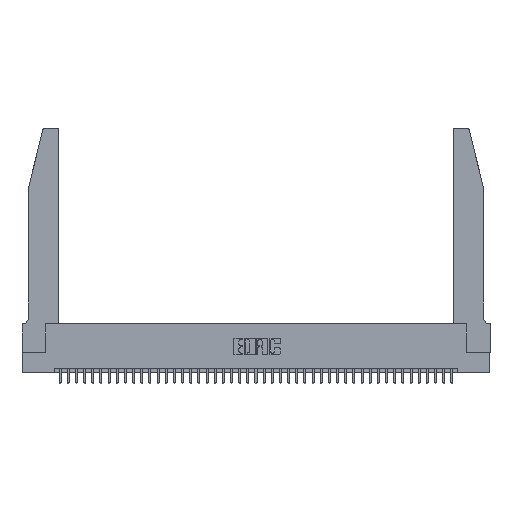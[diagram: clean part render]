
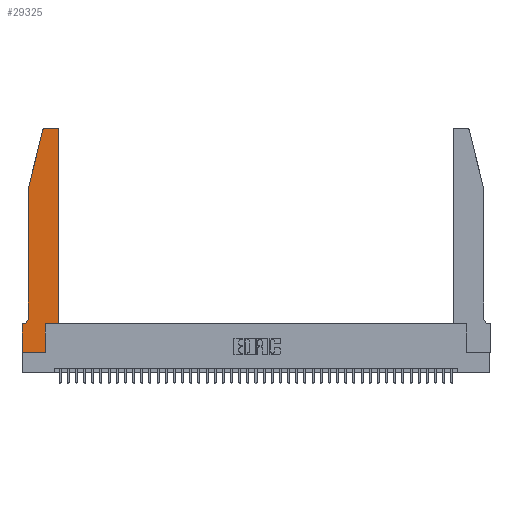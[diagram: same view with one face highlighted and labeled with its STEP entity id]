
A CAD part, top view. The second image highlights one B-rep face of the part: STEP entity #29325.
In plain terms, the highlighted planar face has unit normal (0, 0, 1).
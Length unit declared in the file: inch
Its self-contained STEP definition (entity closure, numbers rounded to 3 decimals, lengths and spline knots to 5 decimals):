
#1261 = DIRECTION ( 'NONE',  ( -1., 0., 0. ) ) ;
#1499 = DIRECTION ( 'NONE',  ( 0., 0., 1. ) ) ;
#2262 = DIRECTION ( 'NONE',  ( 1., 0., 0. ) ) ;
#2584 = CARTESIAN_POINT ( 'NONE',  ( 0.25487, 2.72718, 0.37 ) ) ;
#3293 = CARTESIAN_POINT ( 'NONE',  ( 0., 0.35, 0.37 ) ) ;
#3625 = EDGE_CURVE ( 'NONE', #10374, #32949, #15056, .T. ) ;
#3972 = CARTESIAN_POINT ( 'NONE',  ( 0.2865, 0.35, 0.37 ) ) ;
#4015 = EDGE_CURVE ( 'NONE', #4853, #9601, #16036, .T. ) ;
#4325 = VERTEX_POINT ( 'NONE', #10144 ) ;
#4494 = DIRECTION ( 'NONE',  ( 0., 0., 1. ) ) ;
#4853 = VERTEX_POINT ( 'NONE', #22454 ) ;
#4887 = VECTOR ( 'NONE', #25808, 39.37008 ) ;
#5277 = DIRECTION ( 'NONE',  ( 0., 1., 0. ) ) ;
#5725 = ORIENTED_EDGE ( 'NONE', *, *, #22349, .T. ) ;
#7347 = CARTESIAN_POINT ( 'NONE',  ( 0.2605, 2.75, 0.37 ) ) ;
#8233 = ORIENTED_EDGE ( 'NONE', *, *, #22009, .T. ) ;
#8640 = EDGE_CURVE ( 'NONE', #4325, #30004, #28037, .T. ) ;
#9000 = VERTEX_POINT ( 'NONE', #16474 ) ;
#9601 = VERTEX_POINT ( 'NONE', #3972 ) ;
#10123 = CIRCLE ( 'NONE', #16179, 0.07 ) ;
#10144 = CARTESIAN_POINT ( 'NONE',  ( 0.4505, 2.72, 0.37 ) ) ;
#10374 = VERTEX_POINT ( 'NONE', #34008 ) ;
#10415 = EDGE_CURVE ( 'NONE', #10629, #10374, #13049, .T. ) ;
#10629 = VERTEX_POINT ( 'NONE', #2584 ) ;
#10981 = CARTESIAN_POINT ( 'NONE',  ( 0., 0.35, 0.37 ) ) ;
#12049 = VECTOR ( 'NONE', #27769, 39.37008 ) ;
#12278 = VECTOR ( 'NONE', #17100, 39.37008 ) ;
#12733 = EDGE_CURVE ( 'NONE', #9000, #32419, #14911, .T. ) ;
#12800 = ORIENTED_EDGE ( 'NONE', *, *, #36486, .T. ) ;
#13049 = LINE ( 'NONE', #37496, #12049 ) ;
#13916 = CARTESIAN_POINT ( 'NONE',  ( 0., 0., 0.37 ) ) ;
#14637 = CARTESIAN_POINT ( 'NONE',  ( 0., 0., 0.37 ) ) ;
#14911 = LINE ( 'NONE', #40177, #40826 ) ;
#15056 = LINE ( 'NONE', #39338, #39942 ) ;
#15659 = CARTESIAN_POINT ( 'NONE',  ( 0.0755, 0.42, 0.37 ) ) ;
#15841 = CARTESIAN_POINT ( 'NONE',  ( 0.4505, 0.35, 0.37 ) ) ;
#16036 = LINE ( 'NONE', #37938, #40931 ) ;
#16179 = AXIS2_PLACEMENT_3D ( 'NONE', #40415, #21040, #1261 ) ;
#16474 = CARTESIAN_POINT ( 'NONE',  ( 0.0055, 0.35, 0.37 ) ) ;
#16706 = VERTEX_POINT ( 'NONE', #14637 ) ;
#16753 = EDGE_CURVE ( 'NONE', #16706, #4853, #18597, .T. ) ;
#17100 = DIRECTION ( 'NONE',  ( 0., -1., 0. ) ) ;
#18597 = LINE ( 'NONE', #21414, #27311 ) ;
#18947 = AXIS2_PLACEMENT_3D ( 'NONE', #41367, #22028, #2262 ) ;
#19148 = DIRECTION ( 'NONE',  ( 1., 0., 0. ) ) ;
#19918 = DIRECTION ( 'NONE',  ( 0., -1., 0. ) ) ;
#20848 = ORIENTED_EDGE ( 'NONE', *, *, #4015, .T. ) ;
#21040 = DIRECTION ( 'NONE',  ( 0., 0., -1. ) ) ;
#21270 = CARTESIAN_POINT ( 'NONE',  ( 0.4205, 2.72, 0.37 ) ) ;
#21414 = CARTESIAN_POINT ( 'NONE',  ( 0., 0., 0.37 ) ) ;
#22009 = EDGE_CURVE ( 'NONE', #32949, #9000, #10123, .T. ) ;
#22028 = DIRECTION ( 'NONE',  ( 0., 0., 1. ) ) ;
#22349 = EDGE_CURVE ( 'NONE', #9601, #31543, #40097, .T. ) ;
#22454 = CARTESIAN_POINT ( 'NONE',  ( 0.2865, 0., 0.37 ) ) ;
#22950 = VECTOR ( 'NONE', #19148, 39.37008 ) ;
#23155 = VERTEX_POINT ( 'NONE', #32952 ) ;
#24100 = DIRECTION ( 'NONE',  ( -1., 0., 0. ) ) ;
#24577 = DIRECTION ( 'NONE',  ( 1., 0., 0. ) ) ;
#25391 = EDGE_LOOP ( 'NONE', ( #12800, #41317, #27601, #28607, #8233, #38602, #38205, #30024, #20848, #5725, #31524, #40453 ) ) ;
#25808 = DIRECTION ( 'NONE',  ( 0., 1., 0. ) ) ;
#26701 = AXIS2_PLACEMENT_3D ( 'NONE', #21270, #1499, #24577 ) ;
#27311 = VECTOR ( 'NONE', #34362, 39.37008 ) ;
#27463 = DIRECTION ( 'NONE',  ( 1., 0., 0. ) ) ;
#27601 = ORIENTED_EDGE ( 'NONE', *, *, #10415, .T. ) ;
#27713 = CIRCLE ( 'NONE', #18947, 0.03 ) ;
#27769 = DIRECTION ( 'NONE',  ( -0.239, -0.971, 0. ) ) ;
#27847 = CARTESIAN_POINT ( 'NONE',  ( 0.4205, 2.75, 0.37 ) ) ;
#28037 = CIRCLE ( 'NONE', #26701, 0.03 ) ;
#28607 = ORIENTED_EDGE ( 'NONE', *, *, #3625, .T. ) ;
#29325 = ADVANCED_FACE ( 'NONE', ( #41487 ), #40265, .T. ) ;
#30004 = VERTEX_POINT ( 'NONE', #27847 ) ;
#30024 = ORIENTED_EDGE ( 'NONE', *, *, #16753, .T. ) ;
#30252 = DIRECTION ( 'NONE',  ( -1., 0., 0. ) ) ;
#30933 = CARTESIAN_POINT ( 'NONE',  ( 0.4505, 0.35, 0.37 ) ) ;
#31424 = VECTOR ( 'NONE', #30252, 39.37008 ) ;
#31524 = ORIENTED_EDGE ( 'NONE', *, *, #34971, .T. ) ;
#31543 = VERTEX_POINT ( 'NONE', #30933 ) ;
#32419 = VERTEX_POINT ( 'NONE', #3293 ) ;
#32949 = VERTEX_POINT ( 'NONE', #15659 ) ;
#32952 = CARTESIAN_POINT ( 'NONE',  ( 0.284, 2.75, 0.37 ) ) ;
#34008 = CARTESIAN_POINT ( 'NONE',  ( 0.0755, 2., 0.37 ) ) ;
#34362 = DIRECTION ( 'NONE',  ( 1., 0., 0. ) ) ;
#34971 = EDGE_CURVE ( 'NONE', #31543, #4325, #38577, .T. ) ;
#35568 = CARTESIAN_POINT ( 'NONE',  ( 0.4505, 0.35, 0.37 ) ) ;
#36486 = EDGE_CURVE ( 'NONE', #30004, #23155, #37931, .T. ) ;
#37058 = AXIS2_PLACEMENT_3D ( 'NONE', #10981, #4494, #27463 ) ;
#37496 = CARTESIAN_POINT ( 'NONE',  ( 0.0755, 2., 0.37 ) ) ;
#37931 = LINE ( 'NONE', #7347, #31424 ) ;
#37938 = CARTESIAN_POINT ( 'NONE',  ( 0.2865, 0.35, 0.37 ) ) ;
#38205 = ORIENTED_EDGE ( 'NONE', *, *, #38477, .T. ) ;
#38250 = LINE ( 'NONE', #13916, #12278 ) ;
#38477 = EDGE_CURVE ( 'NONE', #32419, #16706, #38250, .T. ) ;
#38577 = LINE ( 'NONE', #35568, #4887 ) ;
#38602 = ORIENTED_EDGE ( 'NONE', *, *, #12733, .T. ) ;
#39338 = CARTESIAN_POINT ( 'NONE',  ( 0.0755, 2., 0.37 ) ) ;
#39942 = VECTOR ( 'NONE', #19918, 39.37008 ) ;
#40097 = LINE ( 'NONE', #15841, #22950 ) ;
#40177 = CARTESIAN_POINT ( 'NONE',  ( 0.0755, 0.35, 0.37 ) ) ;
#40265 = PLANE ( 'NONE',  #37058 ) ;
#40415 = CARTESIAN_POINT ( 'NONE',  ( 0.0055, 0.42, 0.37 ) ) ;
#40453 = ORIENTED_EDGE ( 'NONE', *, *, #8640, .T. ) ;
#40826 = VECTOR ( 'NONE', #24100, 39.37008 ) ;
#40931 = VECTOR ( 'NONE', #5277, 39.37008 ) ;
#41317 = ORIENTED_EDGE ( 'NONE', *, *, #42206, .T. ) ;
#41367 = CARTESIAN_POINT ( 'NONE',  ( 0.284, 2.72, 0.37 ) ) ;
#41487 = FACE_OUTER_BOUND ( 'NONE', #25391, .T. ) ;
#42206 = EDGE_CURVE ( 'NONE', #23155, #10629, #27713, .T. ) ;
